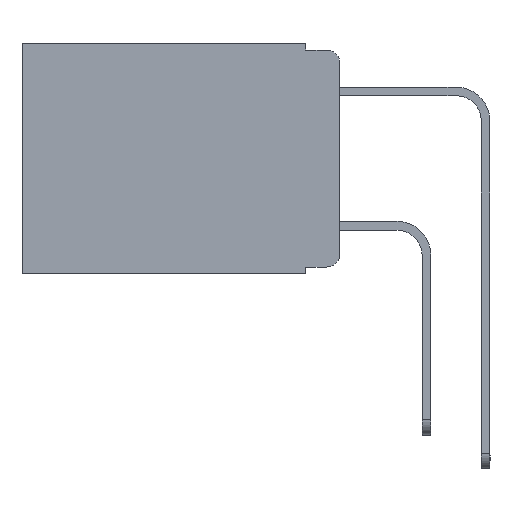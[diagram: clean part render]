
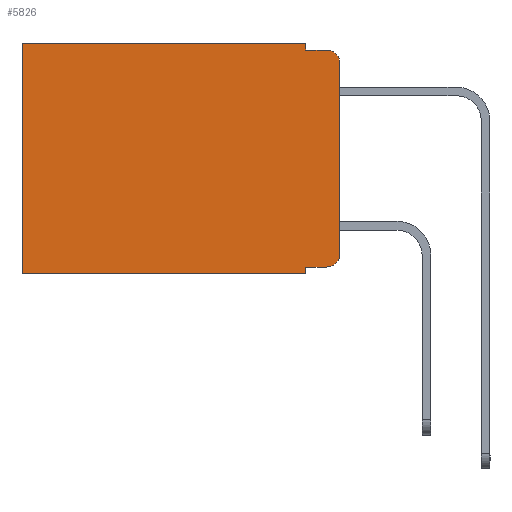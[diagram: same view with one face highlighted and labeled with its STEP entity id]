
A CAD part, left-side view. The second image highlights one B-rep face of the part: STEP entity #5826.
In plain terms, the highlighted planar face has unit normal (-1, 0, 0).
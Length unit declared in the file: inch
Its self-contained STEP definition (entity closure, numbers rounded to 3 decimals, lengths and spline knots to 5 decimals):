
#213 = CARTESIAN_POINT ( 'NONE',  ( 0.298, 0., 0. ) ) ;
#942 = ORIENTED_EDGE ( 'NONE', *, *, #2606, .T. ) ;
#978 = DIRECTION ( 'NONE',  ( 0., 1., 0. ) ) ;
#1000 = EDGE_CURVE ( 'NONE', #5937, #6639, #4956, .T. ) ;
#1043 = VECTOR ( 'NONE', #6211, 39.37008 ) ;
#1308 = ORIENTED_EDGE ( 'NONE', *, *, #20416, .T. ) ;
#1427 = ORIENTED_EDGE ( 'NONE', *, *, #22886, .F. ) ;
#1902 = CARTESIAN_POINT ( 'NONE',  ( 0.298, 0.051, 0. ) ) ;
#2355 = AXIS2_PLACEMENT_3D ( 'NONE', #19792, #11108, #18385 ) ;
#2464 = DIRECTION ( 'NONE',  ( 0., -1., 0. ) ) ;
#2606 = EDGE_CURVE ( 'NONE', #6639, #19790, #15202, .T. ) ;
#2962 = FACE_OUTER_BOUND ( 'NONE', #20662, .T. ) ;
#3460 = VERTEX_POINT ( 'NONE', #22540 ) ;
#3566 = CARTESIAN_POINT ( 'NONE',  ( 0.298, 0.02, -0.01 ) ) ;
#4311 = AXIS2_PLACEMENT_3D ( 'NONE', #22713, #23167, #19417 ) ;
#4746 = LINE ( 'NONE', #9671, #12351 ) ;
#4757 = CARTESIAN_POINT ( 'NONE',  ( 0.298, 0.051, -0.01 ) ) ;
#4814 = CARTESIAN_POINT ( 'NONE',  ( 0.298, 0.02, -0.333 ) ) ;
#4956 = LINE ( 'NONE', #8942, #16493 ) ;
#5329 = CARTESIAN_POINT ( 'NONE',  ( 0.298, 0.473, -0.343 ) ) ;
#5826 = ADVANCED_FACE ( 'NONE', ( #2962 ), #6945, .F. ) ;
#5937 = VERTEX_POINT ( 'NONE', #1902 ) ;
#6211 = DIRECTION ( 'NONE',  ( 0., 0., -1. ) ) ;
#6280 = VERTEX_POINT ( 'NONE', #12204 ) ;
#6639 = VERTEX_POINT ( 'NONE', #17922 ) ;
#6945 = PLANE ( 'NONE',  #4311 ) ;
#7496 = ORIENTED_EDGE ( 'NONE', *, *, #18048, .T. ) ;
#7811 = VECTOR ( 'NONE', #10389, 39.37008 ) ;
#7873 = CARTESIAN_POINT ( 'NONE',  ( 0.298, 0.051, 0. ) ) ;
#7999 = ORIENTED_EDGE ( 'NONE', *, *, #18975, .F. ) ;
#8330 = CARTESIAN_POINT ( 'NONE',  ( 0.298, 0.051, 0. ) ) ;
#8598 = CARTESIAN_POINT ( 'NONE',  ( 0.298, 0.051, -0.333 ) ) ;
#8942 = CARTESIAN_POINT ( 'NONE',  ( 0.298, 0., 0. ) ) ;
#8990 = ORIENTED_EDGE ( 'NONE', *, *, #10796, .F. ) ;
#9597 = DIRECTION ( 'NONE',  ( 0., 0., -1. ) ) ;
#9671 = CARTESIAN_POINT ( 'NONE',  ( 0.298, 0., -0.343 ) ) ;
#10022 = VECTOR ( 'NONE', #2464, 39.37008 ) ;
#10064 = CARTESIAN_POINT ( 'NONE',  ( 0.298, 0., -0.313 ) ) ;
#10234 = DIRECTION ( 'NONE',  ( 0., 0., -1. ) ) ;
#10245 = AXIS2_PLACEMENT_3D ( 'NONE', #22798, #12008, #10234 ) ;
#10281 = VECTOR ( 'NONE', #13076, 39.37008 ) ;
#10389 = DIRECTION ( 'NONE',  ( 0., -1., 0. ) ) ;
#10796 = EDGE_CURVE ( 'NONE', #13416, #6280, #11063, .T. ) ;
#10803 = EDGE_CURVE ( 'NONE', #13416, #13765, #22219, .T. ) ;
#11063 = LINE ( 'NONE', #7873, #17157 ) ;
#11108 = DIRECTION ( 'NONE',  ( -1., 0., 0. ) ) ;
#11309 = ORIENTED_EDGE ( 'NONE', *, *, #12973, .F. ) ;
#11753 = VERTEX_POINT ( 'NONE', #3566 ) ;
#11871 = LINE ( 'NONE', #8330, #1043 ) ;
#11894 = EDGE_CURVE ( 'NONE', #5937, #20254, #11871, .T. ) ;
#12008 = DIRECTION ( 'NONE',  ( -1., 0., 0. ) ) ;
#12204 = CARTESIAN_POINT ( 'NONE',  ( 0.298, 0.051, -0.343 ) ) ;
#12234 = ORIENTED_EDGE ( 'NONE', *, *, #10803, .T. ) ;
#12351 = VECTOR ( 'NONE', #978, 39.37008 ) ;
#12973 = EDGE_CURVE ( 'NONE', #20254, #11753, #17208, .T. ) ;
#13076 = DIRECTION ( 'NONE',  ( 0., 0., -1. ) ) ;
#13416 = VERTEX_POINT ( 'NONE', #8598 ) ;
#13435 = CARTESIAN_POINT ( 'NONE',  ( 0.298, 0.473, 0. ) ) ;
#13765 = VERTEX_POINT ( 'NONE', #4814 ) ;
#14589 = DIRECTION ( 'NONE',  ( 0., 0., -1. ) ) ;
#15202 = LINE ( 'NONE', #13435, #10281 ) ;
#16323 = LINE ( 'NONE', #213, #17006 ) ;
#16493 = VECTOR ( 'NONE', #21169, 39.37008 ) ;
#17006 = VECTOR ( 'NONE', #9597, 39.37008 ) ;
#17157 = VECTOR ( 'NONE', #14589, 39.37008 ) ;
#17208 = LINE ( 'NONE', #4757, #7811 ) ;
#17378 = CIRCLE ( 'NONE', #10245, 0.02 ) ;
#17379 = CIRCLE ( 'NONE', #2355, 0.02 ) ;
#17794 = ORIENTED_EDGE ( 'NONE', *, *, #11894, .F. ) ;
#17922 = CARTESIAN_POINT ( 'NONE',  ( 0.298, 0.473, 0. ) ) ;
#18048 = EDGE_CURVE ( 'NONE', #13765, #19199, #17379, .T. ) ;
#18385 = DIRECTION ( 'NONE',  ( 0., 0., -1. ) ) ;
#18581 = CARTESIAN_POINT ( 'NONE',  ( 0.298, 0.051, -0.333 ) ) ;
#18590 = ORIENTED_EDGE ( 'NONE', *, *, #1000, .T. ) ;
#18975 = EDGE_CURVE ( 'NONE', #3460, #19199, #16323, .T. ) ;
#19199 = VERTEX_POINT ( 'NONE', #10064 ) ;
#19417 = DIRECTION ( 'NONE',  ( 0., 0., -1. ) ) ;
#19790 = VERTEX_POINT ( 'NONE', #5329 ) ;
#19792 = CARTESIAN_POINT ( 'NONE',  ( 0.298, 0.02, -0.313 ) ) ;
#20254 = VERTEX_POINT ( 'NONE', #21762 ) ;
#20416 = EDGE_CURVE ( 'NONE', #3460, #11753, #17378, .T. ) ;
#20662 = EDGE_LOOP ( 'NONE', ( #7999, #1308, #11309, #17794, #18590, #942, #1427, #8990, #12234, #7496 ) ) ;
#21169 = DIRECTION ( 'NONE',  ( 0., 1., 0. ) ) ;
#21762 = CARTESIAN_POINT ( 'NONE',  ( 0.298, 0.051, -0.01 ) ) ;
#22219 = LINE ( 'NONE', #18581, #10022 ) ;
#22540 = CARTESIAN_POINT ( 'NONE',  ( 0.298, 0., -0.03 ) ) ;
#22713 = CARTESIAN_POINT ( 'NONE',  ( 0.298, 0., 0. ) ) ;
#22798 = CARTESIAN_POINT ( 'NONE',  ( 0.298, 0.02, -0.03 ) ) ;
#22886 = EDGE_CURVE ( 'NONE', #6280, #19790, #4746, .T. ) ;
#23167 = DIRECTION ( 'NONE',  ( 1., 0., 0. ) ) ;
